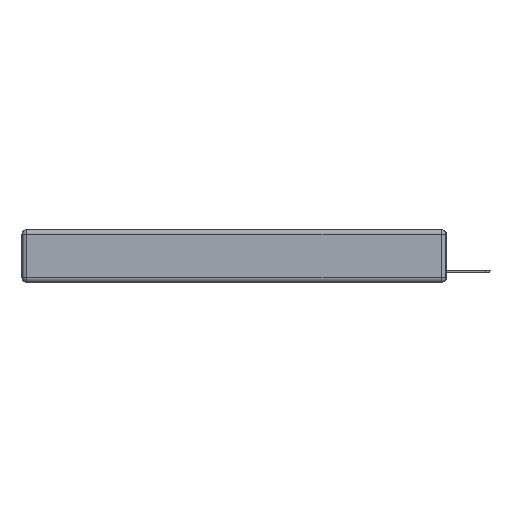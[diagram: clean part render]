
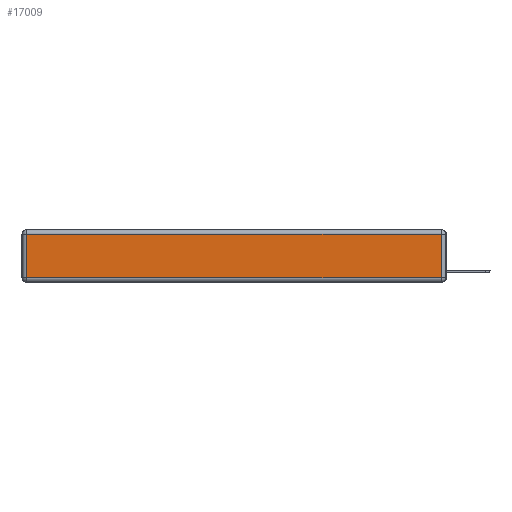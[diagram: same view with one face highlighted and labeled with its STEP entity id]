
A CAD part, left-side view. The second image highlights one B-rep face of the part: STEP entity #17009.
In plain terms, the highlighted planar face has unit normal (-1, 0, 0).
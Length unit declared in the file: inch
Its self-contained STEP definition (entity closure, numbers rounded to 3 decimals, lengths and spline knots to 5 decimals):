
#162 = LINE ( 'NONE', #12454, #712 ) ;
#334 = CARTESIAN_POINT ( 'NONE',  ( 0., 2.72, -0.03 ) ) ;
#712 = VECTOR ( 'NONE', #17546, 39.37008 ) ;
#2069 = DIRECTION ( 'NONE',  ( 0., 0., 1. ) ) ;
#2106 = FACE_OUTER_BOUND ( 'NONE', #12746, .T. ) ;
#3056 = DIRECTION ( 'NONE',  ( 0., 0., 1. ) ) ;
#5218 = EDGE_CURVE ( 'NONE', #20674, #17979, #6128, .T. ) ;
#6128 = LINE ( 'NONE', #13691, #17618 ) ;
#6490 = DIRECTION ( 'NONE',  ( 0., 1., 0. ) ) ;
#6662 = ORIENTED_EDGE ( 'NONE', *, *, #5218, .T. ) ;
#7782 = VERTEX_POINT ( 'NONE', #13269 ) ;
#9337 = CARTESIAN_POINT ( 'NONE',  ( 0., 2.72, -0.343 ) ) ;
#10352 = CARTESIAN_POINT ( 'NONE',  ( 0., 0.03, -0.343 ) ) ;
#10930 = DIRECTION ( 'NONE',  ( -1., 0., 0. ) ) ;
#12085 = EDGE_CURVE ( 'NONE', #21990, #7782, #162, .T. ) ;
#12131 = VECTOR ( 'NONE', #19640, 39.37008 ) ;
#12208 = ORIENTED_EDGE ( 'NONE', *, *, #12085, .T. ) ;
#12436 = LINE ( 'NONE', #10352, #17626 ) ;
#12454 = CARTESIAN_POINT ( 'NONE',  ( 0., 0., -0.313 ) ) ;
#12570 = EDGE_CURVE ( 'NONE', #17979, #21990, #20332, .T. ) ;
#12645 = ORIENTED_EDGE ( 'NONE', *, *, #12570, .T. ) ;
#12746 = EDGE_LOOP ( 'NONE', ( #12208, #17049, #6662, #12645 ) ) ;
#13269 = CARTESIAN_POINT ( 'NONE',  ( 0., 0.03, -0.313 ) ) ;
#13691 = CARTESIAN_POINT ( 'NONE',  ( 0., 2.75, -0.03 ) ) ;
#15289 = CARTESIAN_POINT ( 'NONE',  ( 0., 0.03, -0.03 ) ) ;
#17009 = ADVANCED_FACE ( 'NONE', ( #2106 ), #19543, .T. ) ;
#17049 = ORIENTED_EDGE ( 'NONE', *, *, #18365, .T. ) ;
#17546 = DIRECTION ( 'NONE',  ( 0., -1., 0. ) ) ;
#17618 = VECTOR ( 'NONE', #6490, 39.37008 ) ;
#17626 = VECTOR ( 'NONE', #3056, 39.37008 ) ;
#17979 = VERTEX_POINT ( 'NONE', #334 ) ;
#18365 = EDGE_CURVE ( 'NONE', #7782, #20674, #12436, .T. ) ;
#19543 = PLANE ( 'NONE',  #21885 ) ;
#19640 = DIRECTION ( 'NONE',  ( 0., 0., -1. ) ) ;
#20025 = CARTESIAN_POINT ( 'NONE',  ( 0., 2.72, -0.313 ) ) ;
#20332 = LINE ( 'NONE', #9337, #12131 ) ;
#20674 = VERTEX_POINT ( 'NONE', #15289 ) ;
#21362 = CARTESIAN_POINT ( 'NONE',  ( 0., 0., -0.343 ) ) ;
#21885 = AXIS2_PLACEMENT_3D ( 'NONE', #21362, #10930, #2069 ) ;
#21990 = VERTEX_POINT ( 'NONE', #20025 ) ;
